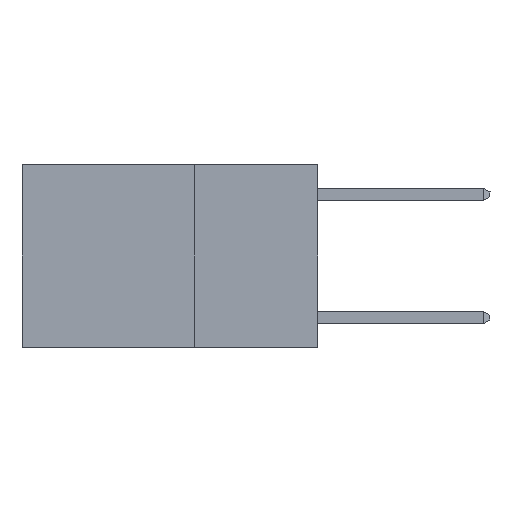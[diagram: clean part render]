
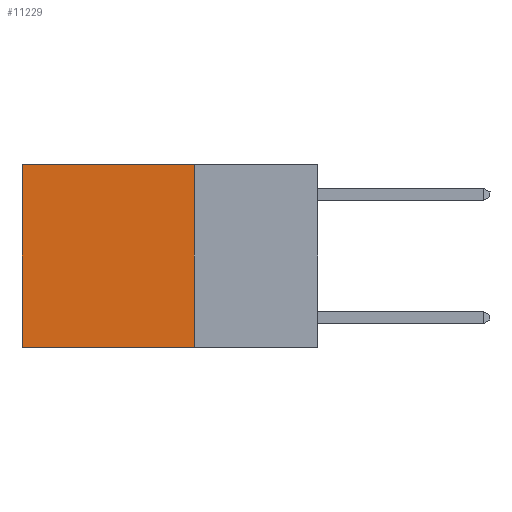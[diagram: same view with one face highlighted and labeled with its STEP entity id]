
A CAD part, left-side view. The second image highlights one B-rep face of the part: STEP entity #11229.
In plain terms, the highlighted planar face has unit normal (-1, 0, 0).
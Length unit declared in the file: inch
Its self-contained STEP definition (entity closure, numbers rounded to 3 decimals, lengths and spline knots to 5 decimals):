
#19 = CARTESIAN_POINT ( 'NONE',  ( 0.2625, 0.6, 0. ) ) ;
#273 = DIRECTION ( 'NONE',  ( 0., 0., -1. ) ) ;
#646 = ORIENTED_EDGE ( 'NONE', *, *, #18659, .F. ) ;
#782 = DIRECTION ( 'NONE',  ( 0., 0., -1. ) ) ;
#1052 = FACE_OUTER_BOUND ( 'NONE', #19349, .T. ) ;
#1200 = LINE ( 'NONE', #15256, #4824 ) ;
#1928 = VECTOR ( 'NONE', #782, 39.37008 ) ;
#2024 = VECTOR ( 'NONE', #10883, 39.37008 ) ;
#2431 = LINE ( 'NONE', #3876, #1928 ) ;
#3876 = CARTESIAN_POINT ( 'NONE',  ( 0.2625, 0.6, 0. ) ) ;
#4824 = VECTOR ( 'NONE', #12992, 39.37008 ) ;
#5302 = ORIENTED_EDGE ( 'NONE', *, *, #14034, .T. ) ;
#6147 = LINE ( 'NONE', #9324, #2024 ) ;
#6417 = PLANE ( 'NONE',  #10464 ) ;
#7396 = VERTEX_POINT ( 'NONE', #17831 ) ;
#7739 = ORIENTED_EDGE ( 'NONE', *, *, #14343, .F. ) ;
#8551 = LINE ( 'NONE', #18600, #16680 ) ;
#9324 = CARTESIAN_POINT ( 'NONE',  ( 0.2625, 0.25, 0. ) ) ;
#9464 = DIRECTION ( 'NONE',  ( 1., 0., 0. ) ) ;
#10464 = AXIS2_PLACEMENT_3D ( 'NONE', #18625, #9464, #273 ) ;
#10883 = DIRECTION ( 'NONE',  ( 0., 1., 0. ) ) ;
#11177 = EDGE_CURVE ( 'NONE', #7396, #19238, #6147, .T. ) ;
#11229 = ADVANCED_FACE ( 'NONE', ( #1052 ), #6417, .F. ) ;
#11562 = CARTESIAN_POINT ( 'NONE',  ( 0.2625, 0.25, -0.37 ) ) ;
#12083 = ORIENTED_EDGE ( 'NONE', *, *, #11177, .T. ) ;
#12312 = VERTEX_POINT ( 'NONE', #19508 ) ;
#12537 = DIRECTION ( 'NONE',  ( 0., 0., -1. ) ) ;
#12992 = DIRECTION ( 'NONE',  ( 0., 1., 0. ) ) ;
#14034 = EDGE_CURVE ( 'NONE', #19238, #12312, #2431, .T. ) ;
#14343 = EDGE_CURVE ( 'NONE', #15378, #12312, #1200, .T. ) ;
#15256 = CARTESIAN_POINT ( 'NONE',  ( 0.2625, 0.25, -0.37 ) ) ;
#15378 = VERTEX_POINT ( 'NONE', #11562 ) ;
#16680 = VECTOR ( 'NONE', #12537, 39.37008 ) ;
#17831 = CARTESIAN_POINT ( 'NONE',  ( 0.2625, 0.25, 0. ) ) ;
#18600 = CARTESIAN_POINT ( 'NONE',  ( 0.2625, 0.25, 0. ) ) ;
#18625 = CARTESIAN_POINT ( 'NONE',  ( 0.2625, 0.25, 0. ) ) ;
#18659 = EDGE_CURVE ( 'NONE', #7396, #15378, #8551, .T. ) ;
#19238 = VERTEX_POINT ( 'NONE', #19 ) ;
#19349 = EDGE_LOOP ( 'NONE', ( #5302, #7739, #646, #12083 ) ) ;
#19508 = CARTESIAN_POINT ( 'NONE',  ( 0.2625, 0.6, -0.37 ) ) ;
